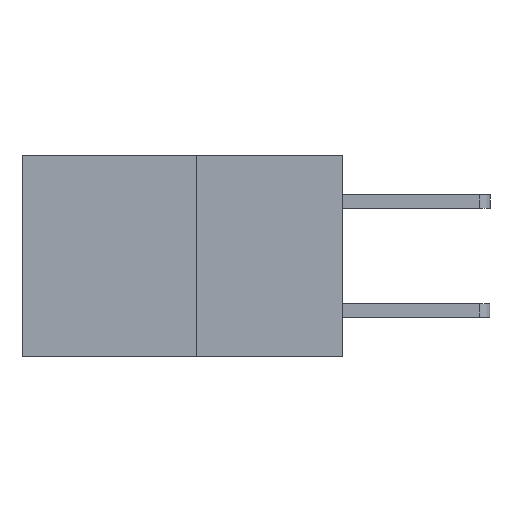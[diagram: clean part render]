
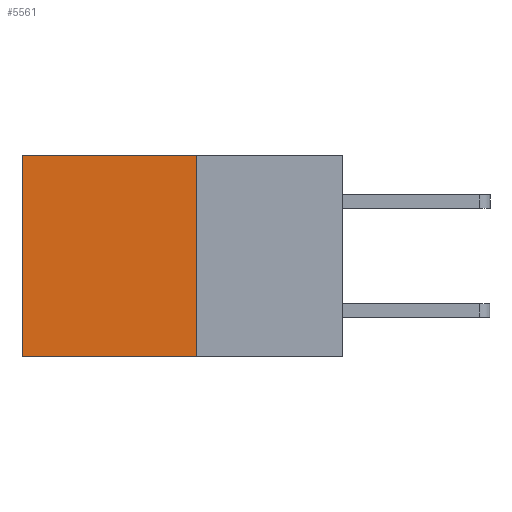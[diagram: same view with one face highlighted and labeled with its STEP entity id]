
A CAD part, left-side view. The second image highlights one B-rep face of the part: STEP entity #5561.
In plain terms, the highlighted planar face has unit normal (-1, 0, 0).
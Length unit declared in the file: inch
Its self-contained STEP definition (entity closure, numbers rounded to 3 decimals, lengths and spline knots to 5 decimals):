
#918 = VERTEX_POINT ( 'NONE', #7452 ) ;
#947 = EDGE_LOOP ( 'NONE', ( #4331, #4300, #3652, #6337 ) ) ;
#1373 = DIRECTION ( 'NONE',  ( 0., 0., -1. ) ) ;
#1941 = VERTEX_POINT ( 'NONE', #3702 ) ;
#1957 = VERTEX_POINT ( 'NONE', #3856 ) ;
#2092 = EDGE_CURVE ( 'NONE', #1957, #918, #4720, .T. ) ;
#2424 = CARTESIAN_POINT ( 'NONE',  ( 0.277, 0.59, -0.37 ) ) ;
#2724 = DIRECTION ( 'NONE',  ( 0., 1., 0. ) ) ;
#2730 = CARTESIAN_POINT ( 'NONE',  ( 0.277, 0.59, -0.37 ) ) ;
#3087 = CARTESIAN_POINT ( 'NONE',  ( 0.277, 0.27, -0.37 ) ) ;
#3225 = EDGE_CURVE ( 'NONE', #1957, #1941, #7017, .T. ) ;
#3652 = ORIENTED_EDGE ( 'NONE', *, *, #3225, .F. ) ;
#3702 = CARTESIAN_POINT ( 'NONE',  ( 0.277, 0.27, -0.37 ) ) ;
#3856 = CARTESIAN_POINT ( 'NONE',  ( 0.277, 0.27, 0. ) ) ;
#3984 = DIRECTION ( 'NONE',  ( 0., 0., -1. ) ) ;
#4243 = VECTOR ( 'NONE', #2724, 39.37008 ) ;
#4250 = FACE_OUTER_BOUND ( 'NONE', #947, .T. ) ;
#4261 = CARTESIAN_POINT ( 'NONE',  ( 0.277, 0.27, -0.37 ) ) ;
#4300 = ORIENTED_EDGE ( 'NONE', *, *, #6558, .F. ) ;
#4324 = CARTESIAN_POINT ( 'NONE',  ( 0.277, 0.27, -0.37 ) ) ;
#4331 = ORIENTED_EDGE ( 'NONE', *, *, #6303, .T. ) ;
#4376 = VECTOR ( 'NONE', #6353, 39.37008 ) ;
#4404 = VERTEX_POINT ( 'NONE', #2424 ) ;
#4720 = LINE ( 'NONE', #5494, #4376 ) ;
#5494 = CARTESIAN_POINT ( 'NONE',  ( 0.277, 0.27, 0. ) ) ;
#5561 = ADVANCED_FACE ( 'NONE', ( #4250 ), #6379, .F. ) ;
#5592 = VECTOR ( 'NONE', #1373, 39.37008 ) ;
#6164 = LINE ( 'NONE', #2730, #7419 ) ;
#6303 = EDGE_CURVE ( 'NONE', #918, #4404, #6164, .T. ) ;
#6337 = ORIENTED_EDGE ( 'NONE', *, *, #2092, .T. ) ;
#6353 = DIRECTION ( 'NONE',  ( 0., 1., 0. ) ) ;
#6379 = PLANE ( 'NONE',  #6938 ) ;
#6474 = DIRECTION ( 'NONE',  ( 0., 0., -1. ) ) ;
#6558 = EDGE_CURVE ( 'NONE', #1941, #4404, #7335, .T. ) ;
#6938 = AXIS2_PLACEMENT_3D ( 'NONE', #4324, #7118, #6474 ) ;
#7017 = LINE ( 'NONE', #4261, #5592 ) ;
#7118 = DIRECTION ( 'NONE',  ( 1., 0., 0. ) ) ;
#7335 = LINE ( 'NONE', #3087, #4243 ) ;
#7419 = VECTOR ( 'NONE', #3984, 39.37008 ) ;
#7452 = CARTESIAN_POINT ( 'NONE',  ( 0.277, 0.59, 0. ) ) ;
